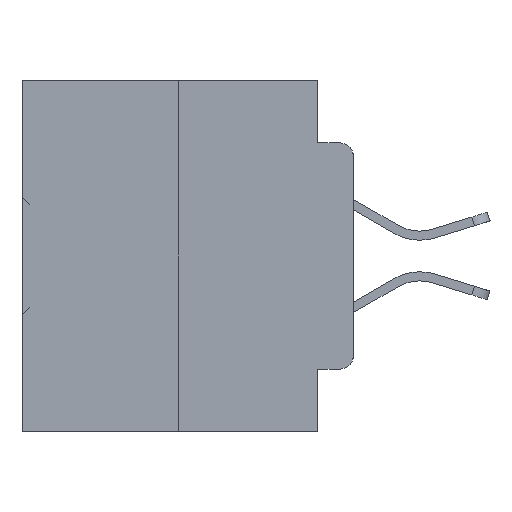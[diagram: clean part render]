
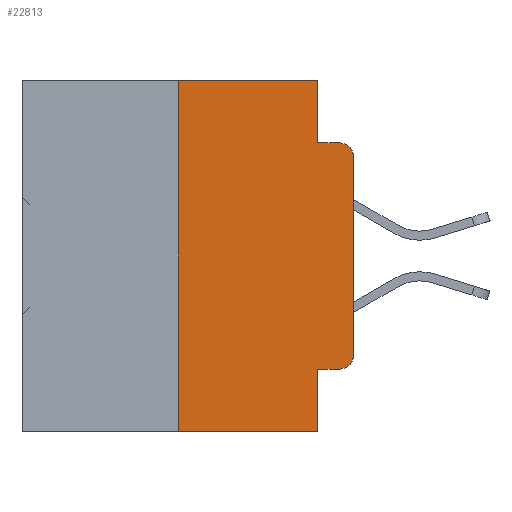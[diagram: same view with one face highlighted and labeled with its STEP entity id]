
A CAD part, left-side view. The second image highlights one B-rep face of the part: STEP entity #22813.
In plain terms, the highlighted planar face has unit normal (-1, 0, 0).
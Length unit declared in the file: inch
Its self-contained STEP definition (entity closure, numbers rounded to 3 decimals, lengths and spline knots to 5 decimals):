
#109 = VERTEX_POINT ( 'NONE', #12856 ) ;
#982 = CARTESIAN_POINT ( 'NONE',  ( 0., 0.051, -0.4115 ) ) ;
#1726 = CARTESIAN_POINT ( 'NONE',  ( 0., 0., 0. ) ) ;
#1838 = ORIENTED_EDGE ( 'NONE', *, *, #3976, .T. ) ;
#1856 = EDGE_CURVE ( 'NONE', #3130, #109, #24776, .T. ) ;
#1994 = LINE ( 'NONE', #8873, #3869 ) ;
#3130 = VERTEX_POINT ( 'NONE', #10860 ) ;
#3311 = AXIS2_PLACEMENT_3D ( 'NONE', #23105, #29227, #38391 ) ;
#3833 = AXIS2_PLACEMENT_3D ( 'NONE', #23909, #8496, #32984 ) ;
#3869 = VECTOR ( 'NONE', #36115, 39.37008 ) ;
#3976 = EDGE_CURVE ( 'NONE', #28344, #3130, #10314, .T. ) ;
#4511 = CIRCLE ( 'NONE', #3311, 0.02 ) ;
#4714 = VERTEX_POINT ( 'NONE', #19571 ) ;
#5058 = CARTESIAN_POINT ( 'NONE',  ( 0., 0.25, 0. ) ) ;
#5332 = DIRECTION ( 'NONE',  ( 0., 0., -1. ) ) ;
#5443 = PLANE ( 'NONE',  #3833 ) ;
#6652 = VECTOR ( 'NONE', #14087, 39.37008 ) ;
#7476 = CARTESIAN_POINT ( 'NONE',  ( 0., 0.051, -0.4115 ) ) ;
#7531 = VERTEX_POINT ( 'NONE', #37958 ) ;
#7572 = VERTEX_POINT ( 'NONE', #34911 ) ;
#7603 = LINE ( 'NONE', #5058, #6652 ) ;
#7710 = VECTOR ( 'NONE', #37315, 39.37008 ) ;
#8496 = DIRECTION ( 'NONE',  ( 1., 0., 0. ) ) ;
#8873 = CARTESIAN_POINT ( 'NONE',  ( 0., 0.473, 0. ) ) ;
#9699 = EDGE_CURVE ( 'NONE', #28344, #7531, #25122, .T. ) ;
#10213 = EDGE_CURVE ( 'NONE', #109, #32405, #17055, .T. ) ;
#10314 = LINE ( 'NONE', #7476, #23181 ) ;
#10860 = CARTESIAN_POINT ( 'NONE',  ( 0., 0.02, -0.4115 ) ) ;
#11243 = DIRECTION ( 'NONE',  ( 0., 0., -1. ) ) ;
#12644 = CARTESIAN_POINT ( 'NONE',  ( 0., 0.051, 0. ) ) ;
#12856 = CARTESIAN_POINT ( 'NONE',  ( 0., 0., -0.3915 ) ) ;
#13166 = AXIS2_PLACEMENT_3D ( 'NONE', #24274, #14550, #11243 ) ;
#13386 = CARTESIAN_POINT ( 'NONE',  ( 0., 0.473, -0.5 ) ) ;
#13658 = CARTESIAN_POINT ( 'NONE',  ( 0., 0.25, -0.5 ) ) ;
#14087 = DIRECTION ( 'NONE',  ( 0., 0., 1. ) ) ;
#14436 = ORIENTED_EDGE ( 'NONE', *, *, #28883, .F. ) ;
#14550 = DIRECTION ( 'NONE',  ( -1., 0., 0. ) ) ;
#15140 = VECTOR ( 'NONE', #17959, 39.37008 ) ;
#15179 = ORIENTED_EDGE ( 'NONE', *, *, #10213, .T. ) ;
#16104 = VECTOR ( 'NONE', #16742, 39.37008 ) ;
#16742 = DIRECTION ( 'NONE',  ( 0., 0., 1. ) ) ;
#17055 = LINE ( 'NONE', #1726, #16104 ) ;
#17726 = ORIENTED_EDGE ( 'NONE', *, *, #22499, .T. ) ;
#17915 = EDGE_CURVE ( 'NONE', #24501, #7531, #28628, .T. ) ;
#17959 = DIRECTION ( 'NONE',  ( 0., 0., -1. ) ) ;
#18323 = EDGE_CURVE ( 'NONE', #4714, #30295, #1994, .T. ) ;
#18568 = ORIENTED_EDGE ( 'NONE', *, *, #9699, .F. ) ;
#19571 = CARTESIAN_POINT ( 'NONE',  ( 0., 0.25, 0. ) ) ;
#21156 = CARTESIAN_POINT ( 'NONE',  ( 0., 0.051, 0. ) ) ;
#21421 = CARTESIAN_POINT ( 'NONE',  ( 0., 0., -0.1085 ) ) ;
#22499 = EDGE_CURVE ( 'NONE', #32405, #7572, #4511, .T. ) ;
#22813 = ADVANCED_FACE ( 'NONE', ( #25401 ), #5443, .F. ) ;
#22856 = EDGE_CURVE ( 'NONE', #24648, #7572, #39247, .T. ) ;
#23105 = CARTESIAN_POINT ( 'NONE',  ( 0., 0.02, -0.1085 ) ) ;
#23181 = VECTOR ( 'NONE', #25683, 39.37008 ) ;
#23909 = CARTESIAN_POINT ( 'NONE',  ( 0., 0.473, 0. ) ) ;
#24274 = CARTESIAN_POINT ( 'NONE',  ( 0., 0.02, -0.3915 ) ) ;
#24501 = VERTEX_POINT ( 'NONE', #13658 ) ;
#24648 = VERTEX_POINT ( 'NONE', #35719 ) ;
#24776 = CIRCLE ( 'NONE', #13166, 0.02 ) ;
#25122 = LINE ( 'NONE', #21156, #15140 ) ;
#25401 = FACE_OUTER_BOUND ( 'NONE', #38929, .T. ) ;
#25683 = DIRECTION ( 'NONE',  ( 0., -1., 0. ) ) ;
#27173 = ORIENTED_EDGE ( 'NONE', *, *, #27343, .F. ) ;
#27343 = EDGE_CURVE ( 'NONE', #24501, #4714, #7603, .T. ) ;
#28344 = VERTEX_POINT ( 'NONE', #982 ) ;
#28364 = VECTOR ( 'NONE', #5332, 39.37008 ) ;
#28628 = LINE ( 'NONE', #13386, #7710 ) ;
#28883 = EDGE_CURVE ( 'NONE', #30295, #24648, #30311, .T. ) ;
#29227 = DIRECTION ( 'NONE',  ( -1., 0., 0. ) ) ;
#30161 = CARTESIAN_POINT ( 'NONE',  ( 0., 0.051, -0.0885 ) ) ;
#30295 = VERTEX_POINT ( 'NONE', #12644 ) ;
#30311 = LINE ( 'NONE', #38814, #28364 ) ;
#30419 = DIRECTION ( 'NONE',  ( 0., -1., 0. ) ) ;
#32405 = VERTEX_POINT ( 'NONE', #21421 ) ;
#32742 = ORIENTED_EDGE ( 'NONE', *, *, #17915, .T. ) ;
#32984 = DIRECTION ( 'NONE',  ( 0., 0., -1. ) ) ;
#34911 = CARTESIAN_POINT ( 'NONE',  ( 0., 0.02, -0.0885 ) ) ;
#35414 = VECTOR ( 'NONE', #30419, 39.37008 ) ;
#35719 = CARTESIAN_POINT ( 'NONE',  ( 0., 0.051, -0.0885 ) ) ;
#35884 = ORIENTED_EDGE ( 'NONE', *, *, #18323, .F. ) ;
#36115 = DIRECTION ( 'NONE',  ( 0., -1., 0. ) ) ;
#37315 = DIRECTION ( 'NONE',  ( 0., -1., 0. ) ) ;
#37958 = CARTESIAN_POINT ( 'NONE',  ( 0., 0.051, -0.5 ) ) ;
#38391 = DIRECTION ( 'NONE',  ( 0., 0., -1. ) ) ;
#38511 = ORIENTED_EDGE ( 'NONE', *, *, #1856, .T. ) ;
#38814 = CARTESIAN_POINT ( 'NONE',  ( 0., 0.051, 0. ) ) ;
#38841 = ORIENTED_EDGE ( 'NONE', *, *, #22856, .F. ) ;
#38929 = EDGE_LOOP ( 'NONE', ( #15179, #17726, #38841, #14436, #35884, #27173, #32742, #18568, #1838, #38511 ) ) ;
#39247 = LINE ( 'NONE', #30161, #35414 ) ;
